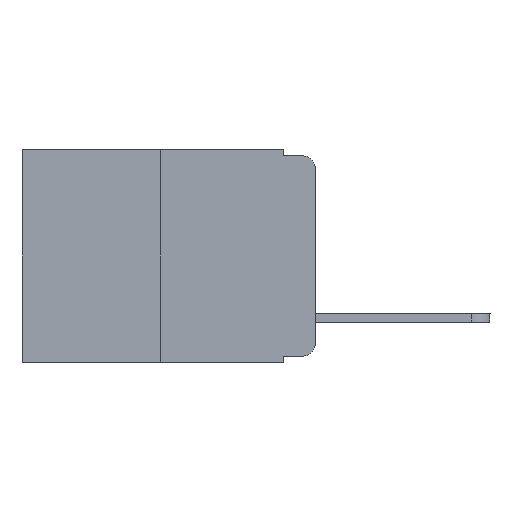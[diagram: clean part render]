
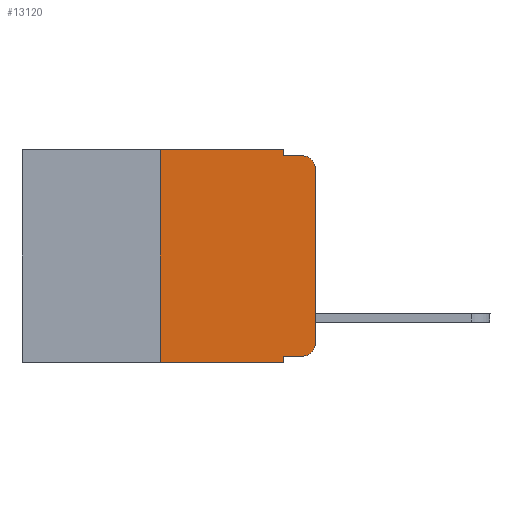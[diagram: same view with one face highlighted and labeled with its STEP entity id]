
A CAD part, left-side view. The second image highlights one B-rep face of the part: STEP entity #13120.
In plain terms, the highlighted planar face has unit normal (-1, 0, 0).
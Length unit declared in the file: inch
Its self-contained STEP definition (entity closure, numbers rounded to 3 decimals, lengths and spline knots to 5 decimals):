
#57 = CIRCLE ( 'NONE', #7664, 0.02 ) ;
#299 = EDGE_CURVE ( 'NONE', #7566, #9617, #4459, .T. ) ;
#647 = DIRECTION ( 'NONE',  ( 0., -1., 0. ) ) ;
#889 = DIRECTION ( 'NONE',  ( 0., 0., -1. ) ) ;
#1062 = CARTESIAN_POINT ( 'NONE',  ( 0., 0.25, 0. ) ) ;
#1101 = EDGE_CURVE ( 'NONE', #3613, #9617, #6648, .T. ) ;
#1116 = DIRECTION ( 'NONE',  ( 0., 0., 1. ) ) ;
#1266 = DIRECTION ( 'NONE',  ( 0., -1., 0. ) ) ;
#1285 = DIRECTION ( 'NONE',  ( 0., 0., 1. ) ) ;
#1314 = CARTESIAN_POINT ( 'NONE',  ( 0., 0.473, -0.343 ) ) ;
#1335 = CARTESIAN_POINT ( 'NONE',  ( 0., 0.02, -0.01 ) ) ;
#1350 = ORIENTED_EDGE ( 'NONE', *, *, #299, .F. ) ;
#1505 = CARTESIAN_POINT ( 'NONE',  ( 0., 0.02, -0.03 ) ) ;
#1733 = VERTEX_POINT ( 'NONE', #4646 ) ;
#1942 = VERTEX_POINT ( 'NONE', #1335 ) ;
#2722 = CARTESIAN_POINT ( 'NONE',  ( 0., 0.051, -0.333 ) ) ;
#3069 = EDGE_LOOP ( 'NONE', ( #13622, #11873, #5238, #3450, #8469, #7955, #5201, #1350, #9902, #3479 ) ) ;
#3245 = VECTOR ( 'NONE', #7094, 39.37008 ) ;
#3383 = LINE ( 'NONE', #14332, #6138 ) ;
#3450 = ORIENTED_EDGE ( 'NONE', *, *, #11506, .F. ) ;
#3479 = ORIENTED_EDGE ( 'NONE', *, *, #14234, .T. ) ;
#3609 = EDGE_CURVE ( 'NONE', #7566, #9696, #3945, .T. ) ;
#3613 = VERTEX_POINT ( 'NONE', #4914 ) ;
#3945 = LINE ( 'NONE', #2722, #3245 ) ;
#3966 = CIRCLE ( 'NONE', #7173, 0.02 ) ;
#4011 = CARTESIAN_POINT ( 'NONE',  ( 0., 0., -0.03 ) ) ;
#4067 = DIRECTION ( 'NONE',  ( -1., 0., 0. ) ) ;
#4128 = VERTEX_POINT ( 'NONE', #1062 ) ;
#4165 = VERTEX_POINT ( 'NONE', #6693 ) ;
#4187 = CARTESIAN_POINT ( 'NONE',  ( 0., 0.473, 0. ) ) ;
#4335 = LINE ( 'NONE', #10944, #12014 ) ;
#4459 = LINE ( 'NONE', #13502, #5811 ) ;
#4603 = EDGE_CURVE ( 'NONE', #9037, #5658, #13136, .T. ) ;
#4646 = CARTESIAN_POINT ( 'NONE',  ( 0., 0.051, 0. ) ) ;
#4678 = CARTESIAN_POINT ( 'NONE',  ( 0., 0.051, -0.333 ) ) ;
#4914 = CARTESIAN_POINT ( 'NONE',  ( 0., 0.25, -0.343 ) ) ;
#4951 = EDGE_CURVE ( 'NONE', #4165, #1942, #5792, .T. ) ;
#4952 = EDGE_CURVE ( 'NONE', #3613, #4128, #3383, .T. ) ;
#5201 = ORIENTED_EDGE ( 'NONE', *, *, #1101, .T. ) ;
#5238 = ORIENTED_EDGE ( 'NONE', *, *, #4951, .F. ) ;
#5658 = VERTEX_POINT ( 'NONE', #4011 ) ;
#5792 = LINE ( 'NONE', #8824, #6365 ) ;
#5811 = VECTOR ( 'NONE', #13285, 39.37008 ) ;
#6138 = VECTOR ( 'NONE', #1116, 39.37008 ) ;
#6210 = LINE ( 'NONE', #6283, #12959 ) ;
#6283 = CARTESIAN_POINT ( 'NONE',  ( 0., 0.473, 0. ) ) ;
#6365 = VECTOR ( 'NONE', #1266, 39.37008 ) ;
#6648 = LINE ( 'NONE', #1314, #11917 ) ;
#6693 = CARTESIAN_POINT ( 'NONE',  ( 0., 0.051, -0.01 ) ) ;
#7094 = DIRECTION ( 'NONE',  ( 0., -1., 0. ) ) ;
#7173 = AXIS2_PLACEMENT_3D ( 'NONE', #10799, #4067, #889 ) ;
#7298 = CARTESIAN_POINT ( 'NONE',  ( 0., 0., -0.313 ) ) ;
#7566 = VERTEX_POINT ( 'NONE', #4678 ) ;
#7664 = AXIS2_PLACEMENT_3D ( 'NONE', #1505, #11357, #12367 ) ;
#7686 = CARTESIAN_POINT ( 'NONE',  ( 0., 0., 0. ) ) ;
#7955 = ORIENTED_EDGE ( 'NONE', *, *, #4952, .F. ) ;
#8469 = ORIENTED_EDGE ( 'NONE', *, *, #9051, .F. ) ;
#8708 = DIRECTION ( 'NONE',  ( 0., 0., -1. ) ) ;
#8796 = DIRECTION ( 'NONE',  ( 0., -1., 0. ) ) ;
#8824 = CARTESIAN_POINT ( 'NONE',  ( 0., 0.051, -0.01 ) ) ;
#8865 = DIRECTION ( 'NONE',  ( 0., 0., -1. ) ) ;
#9037 = VERTEX_POINT ( 'NONE', #7298 ) ;
#9051 = EDGE_CURVE ( 'NONE', #4128, #1733, #6210, .T. ) ;
#9374 = EDGE_CURVE ( 'NONE', #5658, #1942, #57, .T. ) ;
#9617 = VERTEX_POINT ( 'NONE', #11335 ) ;
#9679 = AXIS2_PLACEMENT_3D ( 'NONE', #4187, #9720, #8708 ) ;
#9696 = VERTEX_POINT ( 'NONE', #10072 ) ;
#9720 = DIRECTION ( 'NONE',  ( 1., 0., 0. ) ) ;
#9902 = ORIENTED_EDGE ( 'NONE', *, *, #3609, .T. ) ;
#10072 = CARTESIAN_POINT ( 'NONE',  ( 0., 0.02, -0.333 ) ) ;
#10799 = CARTESIAN_POINT ( 'NONE',  ( 0., 0.02, -0.313 ) ) ;
#10944 = CARTESIAN_POINT ( 'NONE',  ( 0., 0.051, 0. ) ) ;
#11335 = CARTESIAN_POINT ( 'NONE',  ( 0., 0.051, -0.343 ) ) ;
#11357 = DIRECTION ( 'NONE',  ( -1., 0., 0. ) ) ;
#11506 = EDGE_CURVE ( 'NONE', #1733, #4165, #4335, .T. ) ;
#11873 = ORIENTED_EDGE ( 'NONE', *, *, #9374, .T. ) ;
#11917 = VECTOR ( 'NONE', #8796, 39.37008 ) ;
#12014 = VECTOR ( 'NONE', #8865, 39.37008 ) ;
#12162 = FACE_OUTER_BOUND ( 'NONE', #3069, .T. ) ;
#12367 = DIRECTION ( 'NONE',  ( 0., 0., -1. ) ) ;
#12845 = VECTOR ( 'NONE', #1285, 39.37008 ) ;
#12959 = VECTOR ( 'NONE', #647, 39.37008 ) ;
#13120 = ADVANCED_FACE ( 'NONE', ( #12162 ), #13288, .F. ) ;
#13136 = LINE ( 'NONE', #7686, #12845 ) ;
#13285 = DIRECTION ( 'NONE',  ( 0., 0., -1. ) ) ;
#13288 = PLANE ( 'NONE',  #9679 ) ;
#13502 = CARTESIAN_POINT ( 'NONE',  ( 0., 0.051, 0. ) ) ;
#13622 = ORIENTED_EDGE ( 'NONE', *, *, #4603, .T. ) ;
#14234 = EDGE_CURVE ( 'NONE', #9696, #9037, #3966, .T. ) ;
#14332 = CARTESIAN_POINT ( 'NONE',  ( 0., 0.25, 0. ) ) ;
